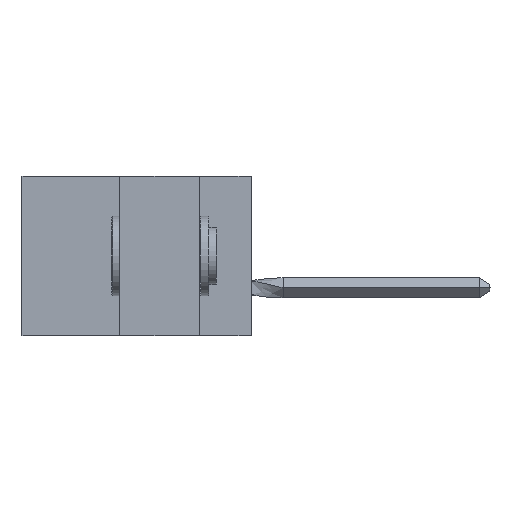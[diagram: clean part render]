
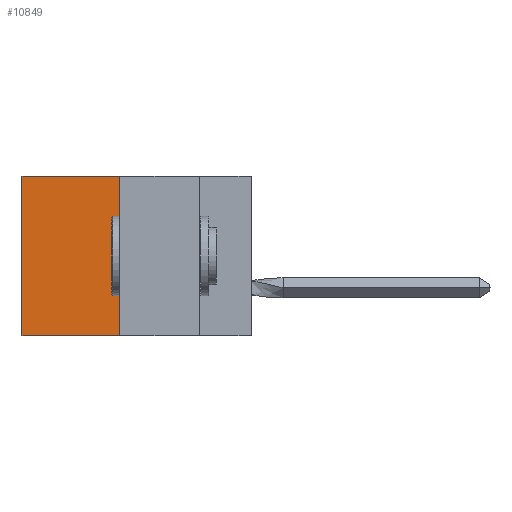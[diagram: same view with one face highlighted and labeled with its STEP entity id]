
A CAD part, left-side view. The second image highlights one B-rep face of the part: STEP entity #10849.
In plain terms, the highlighted planar face has unit normal (-1, 0, 0).
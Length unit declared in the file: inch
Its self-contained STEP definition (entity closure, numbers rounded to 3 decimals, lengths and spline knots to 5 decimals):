
#24 = EDGE_CURVE ( 'NONE', #15293, #14628, #1775, .T. ) ;
#387 = VECTOR ( 'NONE', #12532, 39.37008 ) ;
#443 = ORIENTED_EDGE ( 'NONE', *, *, #14627, .F. ) ;
#753 = EDGE_LOOP ( 'NONE', ( #2993, #17113, #443, #8218 ) ) ;
#842 = AXIS2_PLACEMENT_3D ( 'NONE', #8084, #9491, #12294 ) ;
#1775 = LINE ( 'NONE', #4107, #17641 ) ;
#2484 = CARTESIAN_POINT ( 'NONE',  ( 0.305, 0.413, -0.5 ) ) ;
#2613 = DIRECTION ( 'NONE',  ( 0., 0., -1. ) ) ;
#2993 = ORIENTED_EDGE ( 'NONE', *, *, #24, .T. ) ;
#4107 = CARTESIAN_POINT ( 'NONE',  ( 0.305, 0.72, -0.5 ) ) ;
#4557 = CARTESIAN_POINT ( 'NONE',  ( 0.305, 0.413, 0. ) ) ;
#5231 = DIRECTION ( 'NONE',  ( 0., 1., 0. ) ) ;
#5896 = EDGE_CURVE ( 'NONE', #7933, #15293, #6406, .T. ) ;
#6406 = LINE ( 'NONE', #10896, #13470 ) ;
#7580 = VERTEX_POINT ( 'NONE', #2484 ) ;
#7852 = LINE ( 'NONE', #9685, #387 ) ;
#7933 = VERTEX_POINT ( 'NONE', #4557 ) ;
#8084 = CARTESIAN_POINT ( 'NONE',  ( 0.305, 0.413, -0.5 ) ) ;
#8218 = ORIENTED_EDGE ( 'NONE', *, *, #5896, .T. ) ;
#8263 = CARTESIAN_POINT ( 'NONE',  ( 0.305, 0.413, -0.5 ) ) ;
#8523 = VECTOR ( 'NONE', #11096, 39.37008 ) ;
#9491 = DIRECTION ( 'NONE',  ( 1., 0., 0. ) ) ;
#9685 = CARTESIAN_POINT ( 'NONE',  ( 0.305, 0.413, -0.5 ) ) ;
#10849 = ADVANCED_FACE ( 'NONE', ( #13492 ), #10859, .F. ) ;
#10859 = PLANE ( 'NONE',  #842 ) ;
#10896 = CARTESIAN_POINT ( 'NONE',  ( 0.305, 0.413, 0. ) ) ;
#10965 = CARTESIAN_POINT ( 'NONE',  ( 0.305, 0.72, -0.5 ) ) ;
#11096 = DIRECTION ( 'NONE',  ( 0., 1., 0. ) ) ;
#12294 = DIRECTION ( 'NONE',  ( 0., 0., -1. ) ) ;
#12532 = DIRECTION ( 'NONE',  ( 0., 0., -1. ) ) ;
#13470 = VECTOR ( 'NONE', #5231, 39.37008 ) ;
#13492 = FACE_OUTER_BOUND ( 'NONE', #753, .T. ) ;
#14457 = EDGE_CURVE ( 'NONE', #7580, #14628, #18241, .T. ) ;
#14627 = EDGE_CURVE ( 'NONE', #7933, #7580, #7852, .T. ) ;
#14628 = VERTEX_POINT ( 'NONE', #10965 ) ;
#15293 = VERTEX_POINT ( 'NONE', #15794 ) ;
#15794 = CARTESIAN_POINT ( 'NONE',  ( 0.305, 0.72, 0. ) ) ;
#17113 = ORIENTED_EDGE ( 'NONE', *, *, #14457, .F. ) ;
#17641 = VECTOR ( 'NONE', #2613, 39.37008 ) ;
#18241 = LINE ( 'NONE', #8263, #8523 ) ;
